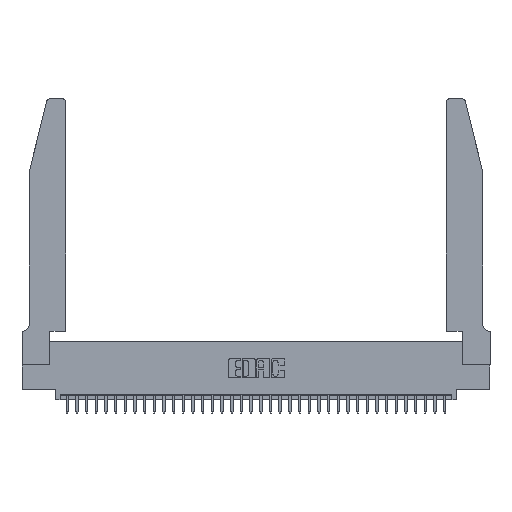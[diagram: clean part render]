
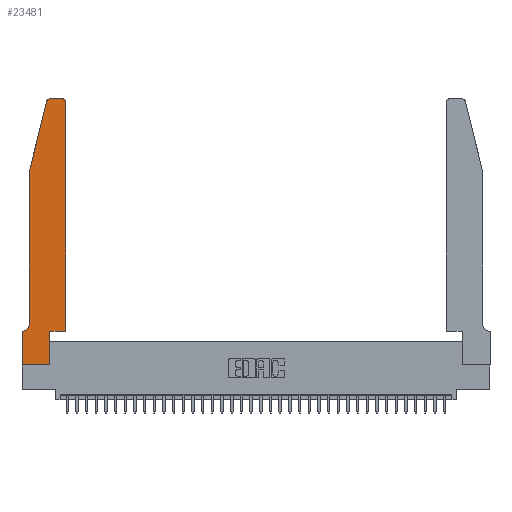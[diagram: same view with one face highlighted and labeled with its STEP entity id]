
A CAD part, top view. The second image highlights one B-rep face of the part: STEP entity #23481.
In plain terms, the highlighted planar face has unit normal (0, 0, 1).
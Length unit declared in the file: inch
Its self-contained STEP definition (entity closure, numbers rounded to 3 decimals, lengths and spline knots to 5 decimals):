
#92 = ORIENTED_EDGE ( 'NONE', *, *, #3156, .T. ) ;
#138 = DIRECTION ( 'NONE',  ( 0., 0., 1. ) ) ;
#273 = VERTEX_POINT ( 'NONE', #24894 ) ;
#338 = ORIENTED_EDGE ( 'NONE', *, *, #36365, .T. ) ;
#587 = CARTESIAN_POINT ( 'NONE',  ( 0.0755, 2., 0.37 ) ) ;
#613 = VERTEX_POINT ( 'NONE', #16315 ) ;
#806 = CARTESIAN_POINT ( 'NONE',  ( 0.4205, 2.72, 0.37 ) ) ;
#1215 = CARTESIAN_POINT ( 'NONE',  ( 0.0755, 0.42, 0.37 ) ) ;
#1587 = ORIENTED_EDGE ( 'NONE', *, *, #32504, .T. ) ;
#2665 = DIRECTION ( 'NONE',  ( 1., 0., 0. ) ) ;
#3156 = EDGE_CURVE ( 'NONE', #21306, #33315, #34768, .T. ) ;
#3508 = LINE ( 'NONE', #587, #8887 ) ;
#3783 = CARTESIAN_POINT ( 'NONE',  ( 0., 0.35, 0.37 ) ) ;
#4221 = CARTESIAN_POINT ( 'NONE',  ( 0., 0., 0.37 ) ) ;
#4439 = ORIENTED_EDGE ( 'NONE', *, *, #35819, .T. ) ;
#5881 = LINE ( 'NONE', #28338, #28790 ) ;
#6770 = VECTOR ( 'NONE', #19509, 39.37008 ) ;
#6958 = VECTOR ( 'NONE', #10741, 39.37008 ) ;
#7097 = VERTEX_POINT ( 'NONE', #32204 ) ;
#7249 = DIRECTION ( 'NONE',  ( -0.239, -0.971, 0. ) ) ;
#7309 = ORIENTED_EDGE ( 'NONE', *, *, #27598, .T. ) ;
#7936 = ORIENTED_EDGE ( 'NONE', *, *, #11737, .T. ) ;
#8493 = LINE ( 'NONE', #15619, #36290 ) ;
#8887 = VECTOR ( 'NONE', #23048, 39.37008 ) ;
#9421 = VECTOR ( 'NONE', #2665, 39.37008 ) ;
#9448 = LINE ( 'NONE', #13852, #6770 ) ;
#9651 = DIRECTION ( 'NONE',  ( 0., 0., 1. ) ) ;
#10437 = AXIS2_PLACEMENT_3D ( 'NONE', #29619, #24243, #13135 ) ;
#10473 = CARTESIAN_POINT ( 'NONE',  ( 0., 0., 0.37 ) ) ;
#10501 = CARTESIAN_POINT ( 'NONE',  ( 0.4505, 0.35, 0.37 ) ) ;
#10648 = CARTESIAN_POINT ( 'NONE',  ( 0., 0., 0.37 ) ) ;
#10741 = DIRECTION ( 'NONE',  ( 0., 1., 0. ) ) ;
#10742 = DIRECTION ( 'NONE',  ( -1., 0., 0. ) ) ;
#11641 = CARTESIAN_POINT ( 'NONE',  ( 0.0055, 0.35, 0.37 ) ) ;
#11737 = EDGE_CURVE ( 'NONE', #32539, #21306, #34554, .T. ) ;
#12086 = PLANE ( 'NONE',  #18720 ) ;
#12149 = EDGE_CURVE ( 'NONE', #32472, #32539, #16011, .T. ) ;
#13135 = DIRECTION ( 'NONE',  ( -1., 0., 0. ) ) ;
#13852 = CARTESIAN_POINT ( 'NONE',  ( 0.2605, 2.75, 0.37 ) ) ;
#14148 = CARTESIAN_POINT ( 'NONE',  ( 0.25487, 2.72718, 0.37 ) ) ;
#14313 = ORIENTED_EDGE ( 'NONE', *, *, #29175, .T. ) ;
#14913 = LINE ( 'NONE', #24901, #34765 ) ;
#14967 = ORIENTED_EDGE ( 'NONE', *, *, #20487, .T. ) ;
#15092 = ORIENTED_EDGE ( 'NONE', *, *, #21194, .T. ) ;
#15619 = CARTESIAN_POINT ( 'NONE',  ( 0.0755, 2., 0.37 ) ) ;
#16011 = LINE ( 'NONE', #10648, #20427 ) ;
#16315 = CARTESIAN_POINT ( 'NONE',  ( 0.4505, 0.35, 0.37 ) ) ;
#17078 = DIRECTION ( 'NONE',  ( 1., 0., 0. ) ) ;
#17989 = DIRECTION ( 'NONE',  ( 1., 0., 0. ) ) ;
#18115 = CARTESIAN_POINT ( 'NONE',  ( 0.284, 2.75, 0.37 ) ) ;
#18720 = AXIS2_PLACEMENT_3D ( 'NONE', #3783, #9651, #17989 ) ;
#18752 = ORIENTED_EDGE ( 'NONE', *, *, #27684, .T. ) ;
#18817 = CARTESIAN_POINT ( 'NONE',  ( 0., 0.35, 0.37 ) ) ;
#19509 = DIRECTION ( 'NONE',  ( -1., 0., 0. ) ) ;
#19584 = CARTESIAN_POINT ( 'NONE',  ( 0.284, 2.72, 0.37 ) ) ;
#20282 = CARTESIAN_POINT ( 'NONE',  ( 0.2865, 0., 0.37 ) ) ;
#20427 = VECTOR ( 'NONE', #30297, 39.37008 ) ;
#20487 = EDGE_CURVE ( 'NONE', #273, #7097, #31032, .T. ) ;
#20511 = ORIENTED_EDGE ( 'NONE', *, *, #29372, .T. ) ;
#20854 = CIRCLE ( 'NONE', #22332, 0.03 ) ;
#21194 = EDGE_CURVE ( 'NONE', #613, #273, #26535, .T. ) ;
#21306 = VERTEX_POINT ( 'NONE', #20282 ) ;
#21407 = ORIENTED_EDGE ( 'NONE', *, *, #12149, .T. ) ;
#22332 = AXIS2_PLACEMENT_3D ( 'NONE', #19584, #138, #17078 ) ;
#22574 = AXIS2_PLACEMENT_3D ( 'NONE', #806, #29212, #29329 ) ;
#23048 = DIRECTION ( 'NONE',  ( 0., -1., 0. ) ) ;
#23481 = ADVANCED_FACE ( 'NONE', ( #28245 ), #12086, .T. ) ;
#23784 = VERTEX_POINT ( 'NONE', #18115 ) ;
#24243 = DIRECTION ( 'NONE',  ( 0., 0., -1. ) ) ;
#24793 = CARTESIAN_POINT ( 'NONE',  ( 0.2865, 0.35, 0.37 ) ) ;
#24894 = CARTESIAN_POINT ( 'NONE',  ( 0.4505, 2.72, 0.37 ) ) ;
#24901 = CARTESIAN_POINT ( 'NONE',  ( 0.0755, 0.35, 0.37 ) ) ;
#25676 = VECTOR ( 'NONE', #28337, 39.37008 ) ;
#25822 = DIRECTION ( 'NONE',  ( 1., 0., 0. ) ) ;
#25852 = VERTEX_POINT ( 'NONE', #14148 ) ;
#25937 = CIRCLE ( 'NONE', #10437, 0.07 ) ;
#26535 = LINE ( 'NONE', #10501, #25676 ) ;
#27576 = CARTESIAN_POINT ( 'NONE',  ( 0.2865, 0.35, 0.37 ) ) ;
#27598 = EDGE_CURVE ( 'NONE', #7097, #23784, #9448, .T. ) ;
#27684 = EDGE_CURVE ( 'NONE', #33315, #613, #5881, .T. ) ;
#28245 = FACE_OUTER_BOUND ( 'NONE', #33869, .T. ) ;
#28337 = DIRECTION ( 'NONE',  ( 0., 1., 0. ) ) ;
#28338 = CARTESIAN_POINT ( 'NONE',  ( 0.4505, 0.35, 0.37 ) ) ;
#28790 = VECTOR ( 'NONE', #25822, 39.37008 ) ;
#29175 = EDGE_CURVE ( 'NONE', #25852, #33893, #8493, .T. ) ;
#29212 = DIRECTION ( 'NONE',  ( 0., 0., 1. ) ) ;
#29329 = DIRECTION ( 'NONE',  ( 1., 0., 0. ) ) ;
#29372 = EDGE_CURVE ( 'NONE', #33893, #29590, #3508, .T. ) ;
#29590 = VERTEX_POINT ( 'NONE', #1215 ) ;
#29619 = CARTESIAN_POINT ( 'NONE',  ( 0.0055, 0.42, 0.37 ) ) ;
#30297 = DIRECTION ( 'NONE',  ( 0., -1., 0. ) ) ;
#31032 = CIRCLE ( 'NONE', #22574, 0.03 ) ;
#32204 = CARTESIAN_POINT ( 'NONE',  ( 0.4205, 2.75, 0.37 ) ) ;
#32472 = VERTEX_POINT ( 'NONE', #18817 ) ;
#32504 = EDGE_CURVE ( 'NONE', #29590, #34185, #25937, .T. ) ;
#32539 = VERTEX_POINT ( 'NONE', #4221 ) ;
#32949 = CARTESIAN_POINT ( 'NONE',  ( 0.0755, 2., 0.37 ) ) ;
#33315 = VERTEX_POINT ( 'NONE', #24793 ) ;
#33869 = EDGE_LOOP ( 'NONE', ( #7309, #4439, #14313, #20511, #1587, #338, #21407, #7936, #92, #18752, #15092, #14967 ) ) ;
#33893 = VERTEX_POINT ( 'NONE', #32949 ) ;
#34185 = VERTEX_POINT ( 'NONE', #11641 ) ;
#34554 = LINE ( 'NONE', #10473, #9421 ) ;
#34765 = VECTOR ( 'NONE', #10742, 39.37008 ) ;
#34768 = LINE ( 'NONE', #27576, #6958 ) ;
#35819 = EDGE_CURVE ( 'NONE', #23784, #25852, #20854, .T. ) ;
#36290 = VECTOR ( 'NONE', #7249, 39.37008 ) ;
#36365 = EDGE_CURVE ( 'NONE', #34185, #32472, #14913, .T. ) ;
